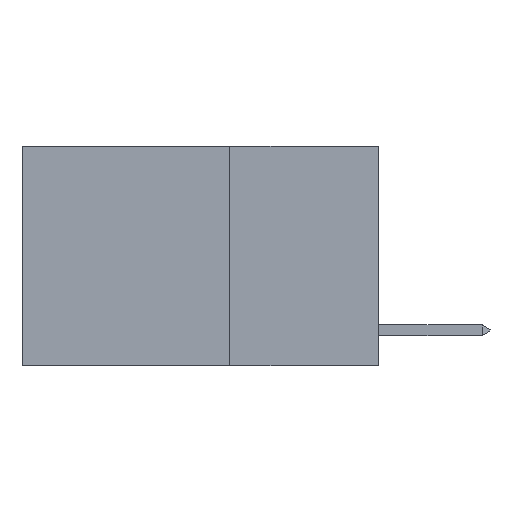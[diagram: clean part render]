
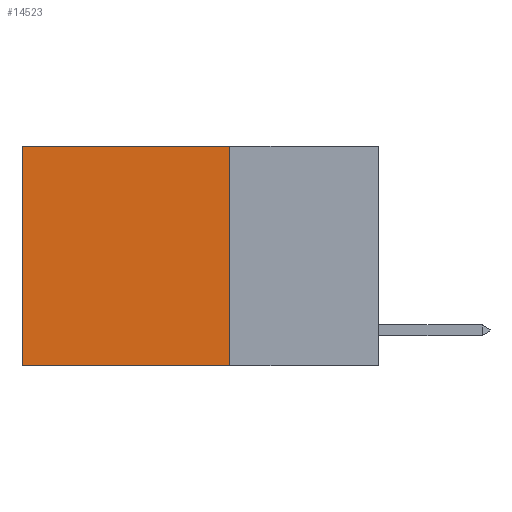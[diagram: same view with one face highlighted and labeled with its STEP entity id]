
A CAD part, left-side view. The second image highlights one B-rep face of the part: STEP entity #14523.
In plain terms, the highlighted planar face has unit normal (-1, 0, 0).
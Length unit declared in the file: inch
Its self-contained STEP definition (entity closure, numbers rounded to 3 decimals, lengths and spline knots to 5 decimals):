
#247 = LINE ( 'NONE', #3458, #12077 ) ;
#1098 = CARTESIAN_POINT ( 'NONE',  ( 0.2625, 0.6, -0.37 ) ) ;
#2283 = ORIENTED_EDGE ( 'NONE', *, *, #9235, .T. ) ;
#2475 = VERTEX_POINT ( 'NONE', #13920 ) ;
#3458 = CARTESIAN_POINT ( 'NONE',  ( 0.2625, 0.25, 0. ) ) ;
#3907 = VECTOR ( 'NONE', #6026, 39.37008 ) ;
#5153 = DIRECTION ( 'NONE',  ( 0., 0., -1. ) ) ;
#5633 = VERTEX_POINT ( 'NONE', #11320 ) ;
#5782 = CARTESIAN_POINT ( 'NONE',  ( 0.2625, 0.25, 0. ) ) ;
#6026 = DIRECTION ( 'NONE',  ( 0., 0., -1. ) ) ;
#6236 = EDGE_CURVE ( 'NONE', #5633, #24745, #25080, .T. ) ;
#7324 = FACE_OUTER_BOUND ( 'NONE', #10056, .T. ) ;
#7769 = PLANE ( 'NONE',  #10454 ) ;
#7850 = DIRECTION ( 'NONE',  ( 1., 0., 0. ) ) ;
#8388 = EDGE_CURVE ( 'NONE', #10030, #5633, #9224, .T. ) ;
#8750 = ORIENTED_EDGE ( 'NONE', *, *, #6236, .F. ) ;
#9172 = LINE ( 'NONE', #11887, #3907 ) ;
#9224 = LINE ( 'NONE', #20933, #24371 ) ;
#9235 = EDGE_CURVE ( 'NONE', #2475, #24745, #9172, .T. ) ;
#10030 = VERTEX_POINT ( 'NONE', #12362 ) ;
#10056 = EDGE_LOOP ( 'NONE', ( #2283, #8750, #24415, #15704 ) ) ;
#10454 = AXIS2_PLACEMENT_3D ( 'NONE', #5782, #7850, #21709 ) ;
#11320 = CARTESIAN_POINT ( 'NONE',  ( 0.2625, 0.25, -0.37 ) ) ;
#11887 = CARTESIAN_POINT ( 'NONE',  ( 0.2625, 0.6, 0. ) ) ;
#12077 = VECTOR ( 'NONE', #17343, 39.37008 ) ;
#12362 = CARTESIAN_POINT ( 'NONE',  ( 0.2625, 0.25, 0. ) ) ;
#13920 = CARTESIAN_POINT ( 'NONE',  ( 0.2625, 0.6, 0. ) ) ;
#14523 = ADVANCED_FACE ( 'NONE', ( #7324 ), #7769, .F. ) ;
#15704 = ORIENTED_EDGE ( 'NONE', *, *, #17664, .T. ) ;
#16421 = DIRECTION ( 'NONE',  ( 0., 1., 0. ) ) ;
#17343 = DIRECTION ( 'NONE',  ( 0., 1., 0. ) ) ;
#17664 = EDGE_CURVE ( 'NONE', #10030, #2475, #247, .T. ) ;
#19884 = VECTOR ( 'NONE', #16421, 39.37008 ) ;
#20933 = CARTESIAN_POINT ( 'NONE',  ( 0.2625, 0.25, 0. ) ) ;
#21709 = DIRECTION ( 'NONE',  ( 0., 0., -1. ) ) ;
#22200 = CARTESIAN_POINT ( 'NONE',  ( 0.2625, 0.25, -0.37 ) ) ;
#24371 = VECTOR ( 'NONE', #5153, 39.37008 ) ;
#24415 = ORIENTED_EDGE ( 'NONE', *, *, #8388, .F. ) ;
#24745 = VERTEX_POINT ( 'NONE', #1098 ) ;
#25080 = LINE ( 'NONE', #22200, #19884 ) ;
